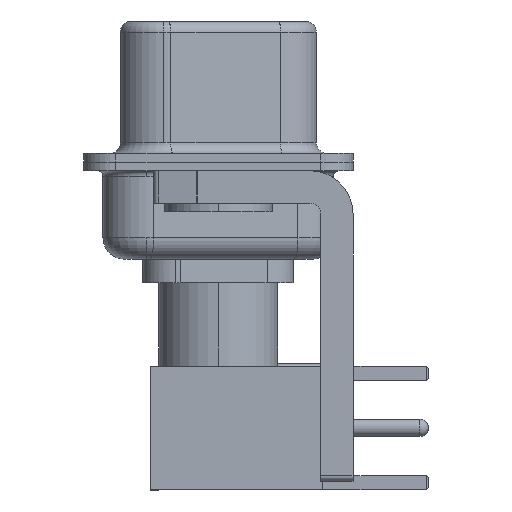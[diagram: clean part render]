
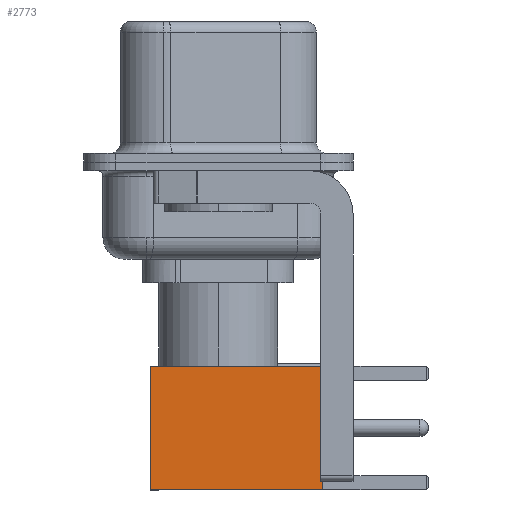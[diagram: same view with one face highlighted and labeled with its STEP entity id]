
A CAD part, left-side view. The second image highlights one B-rep face of the part: STEP entity #2773.
In plain terms, the highlighted face is planar.
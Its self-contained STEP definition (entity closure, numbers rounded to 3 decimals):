
#2490 = DIRECTION ( 'NONE',  ( 0., 0., -1. ) ) ;
#2773 = ADVANCED_FACE ( 'NONE', ( #20354 ), #14962, .T. ) ;
#3329 = EDGE_CURVE ( 'NONE', #10092, #30650, #22971, .T. ) ;
#3665 = ORIENTED_EDGE ( 'NONE', *, *, #26899, .F. ) ;
#4421 = CARTESIAN_POINT ( 'NONE',  ( 2.875, 2.875, 0. ) ) ;
#4595 = EDGE_LOOP ( 'NONE', ( #15254, #27680, #3665, #9458 ) ) ;
#4772 = CARTESIAN_POINT ( 'NONE',  ( 0., 2.875, 8. ) ) ;
#6990 = VECTOR ( 'NONE', #17892, 1000. ) ;
#7798 = DIRECTION ( 'NONE',  ( -1., 0., 0. ) ) ;
#7892 = CARTESIAN_POINT ( 'NONE',  ( 2.875, 2.875, 0. ) ) ;
#9458 = ORIENTED_EDGE ( 'NONE', *, *, #3329, .F. ) ;
#10092 = VERTEX_POINT ( 'NONE', #11859 ) ;
#11859 = CARTESIAN_POINT ( 'NONE',  ( 2.875, 2.875, 8. ) ) ;
#14837 = CARTESIAN_POINT ( 'NONE',  ( 0., 2.875, 0. ) ) ;
#14962 = PLANE ( 'NONE',  #23983 ) ;
#15009 = DIRECTION ( 'NONE',  ( -1., 0., 0. ) ) ;
#15254 = ORIENTED_EDGE ( 'NONE', *, *, #24869, .T. ) ;
#15479 = LINE ( 'NONE', #30812, #29085 ) ;
#17892 = DIRECTION ( 'NONE',  ( 0., 0., -1. ) ) ;
#18176 = VECTOR ( 'NONE', #15009, 1000. ) ;
#18447 = CARTESIAN_POINT ( 'NONE',  ( -2.875, 2.875, 0. ) ) ;
#18691 = VECTOR ( 'NONE', #7798, 1000. ) ;
#19664 = DIRECTION ( 'NONE',  ( 0., 0., 1. ) ) ;
#20354 = FACE_OUTER_BOUND ( 'NONE', #4595, .T. ) ;
#22299 = EDGE_CURVE ( 'NONE', #26956, #25087, #32698, .T. ) ;
#22709 = CARTESIAN_POINT ( 'NONE',  ( 2.875, 2.875, 0. ) ) ;
#22971 = LINE ( 'NONE', #4772, #18691 ) ;
#23983 = AXIS2_PLACEMENT_3D ( 'NONE', #22709, #32986, #19664 ) ;
#24869 = EDGE_CURVE ( 'NONE', #10092, #26956, #33060, .T. ) ;
#25087 = VERTEX_POINT ( 'NONE', #18447 ) ;
#26899 = EDGE_CURVE ( 'NONE', #30650, #25087, #15479, .T. ) ;
#26956 = VERTEX_POINT ( 'NONE', #7892 ) ;
#27680 = ORIENTED_EDGE ( 'NONE', *, *, #22299, .T. ) ;
#29085 = VECTOR ( 'NONE', #2490, 1000. ) ;
#30650 = VERTEX_POINT ( 'NONE', #31459 ) ;
#30812 = CARTESIAN_POINT ( 'NONE',  ( -2.875, 2.875, 0. ) ) ;
#31459 = CARTESIAN_POINT ( 'NONE',  ( -2.875, 2.875, 8. ) ) ;
#32698 = LINE ( 'NONE', #14837, #18176 ) ;
#32986 = DIRECTION ( 'NONE',  ( 0., 1., 0. ) ) ;
#33060 = LINE ( 'NONE', #4421, #6990 ) ;
